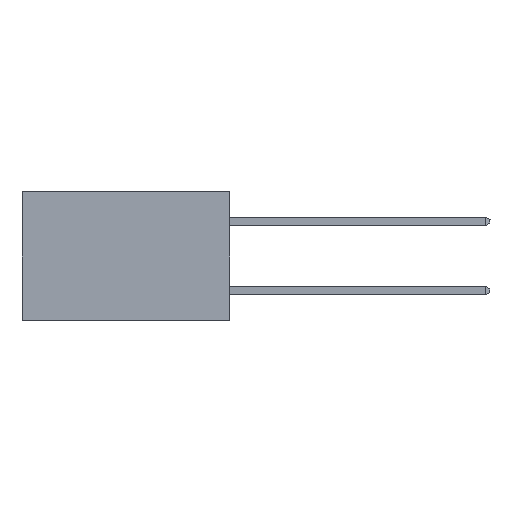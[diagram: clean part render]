
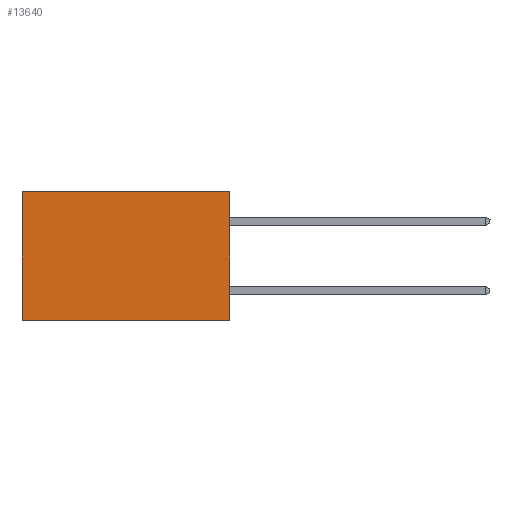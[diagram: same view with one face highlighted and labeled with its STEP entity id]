
A CAD part, left-side view. The second image highlights one B-rep face of the part: STEP entity #13640.
In plain terms, the highlighted planar face has unit normal (-1, 0, 0).
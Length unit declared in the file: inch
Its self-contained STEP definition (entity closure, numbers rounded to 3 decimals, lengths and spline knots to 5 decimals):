
#732 = DIRECTION ( 'NONE',  ( 0., 0., -1. ) ) ;
#771 = ORIENTED_EDGE ( 'NONE', *, *, #5484, .F. ) ;
#996 = VECTOR ( 'NONE', #6871, 39.37008 ) ;
#1110 = CARTESIAN_POINT ( 'NONE',  ( 0.2615, 0.6, -0.37 ) ) ;
#1194 = LINE ( 'NONE', #12657, #16201 ) ;
#1874 = CARTESIAN_POINT ( 'NONE',  ( 0.2615, 0.6, 0. ) ) ;
#2434 = PLANE ( 'NONE',  #10599 ) ;
#3651 = LINE ( 'NONE', #11792, #996 ) ;
#4259 = CARTESIAN_POINT ( 'NONE',  ( 0.2615, 0., -0.37 ) ) ;
#5484 = EDGE_CURVE ( 'NONE', #20255, #8042, #1194, .T. ) ;
#5891 = EDGE_CURVE ( 'NONE', #8042, #10948, #8633, .T. ) ;
#6721 = EDGE_CURVE ( 'NONE', #17228, #10948, #3651, .T. ) ;
#6871 = DIRECTION ( 'NONE',  ( 0., 0., -1. ) ) ;
#8042 = VERTEX_POINT ( 'NONE', #13190 ) ;
#8633 = LINE ( 'NONE', #11843, #10373 ) ;
#9214 = DIRECTION ( 'NONE',  ( 0., 1., 0. ) ) ;
#10373 = VECTOR ( 'NONE', #13558, 39.37008 ) ;
#10599 = AXIS2_PLACEMENT_3D ( 'NONE', #4259, #17211, #732 ) ;
#10783 = ORIENTED_EDGE ( 'NONE', *, *, #6721, .T. ) ;
#10948 = VERTEX_POINT ( 'NONE', #1110 ) ;
#11792 = CARTESIAN_POINT ( 'NONE',  ( 0.2615, 0.6, -0.37 ) ) ;
#11843 = CARTESIAN_POINT ( 'NONE',  ( 0.2615, 0., -0.37 ) ) ;
#11971 = FACE_OUTER_BOUND ( 'NONE', #20858, .T. ) ;
#12657 = CARTESIAN_POINT ( 'NONE',  ( 0.2615, 0., -0.37 ) ) ;
#13190 = CARTESIAN_POINT ( 'NONE',  ( 0.2615, 0., -0.37 ) ) ;
#13197 = EDGE_CURVE ( 'NONE', #20255, #17228, #15544, .T. ) ;
#13558 = DIRECTION ( 'NONE',  ( 0., 1., 0. ) ) ;
#13640 = ADVANCED_FACE ( 'NONE', ( #11971 ), #2434, .F. ) ;
#13858 = CARTESIAN_POINT ( 'NONE',  ( 0.2615, 0., 0. ) ) ;
#14012 = VECTOR ( 'NONE', #9214, 39.37008 ) ;
#15441 = CARTESIAN_POINT ( 'NONE',  ( 0.2615, 0., 0. ) ) ;
#15544 = LINE ( 'NONE', #15441, #14012 ) ;
#16201 = VECTOR ( 'NONE', #19181, 39.37008 ) ;
#17211 = DIRECTION ( 'NONE',  ( 1., 0., 0. ) ) ;
#17228 = VERTEX_POINT ( 'NONE', #1874 ) ;
#18901 = ORIENTED_EDGE ( 'NONE', *, *, #5891, .F. ) ;
#19181 = DIRECTION ( 'NONE',  ( 0., 0., -1. ) ) ;
#19499 = ORIENTED_EDGE ( 'NONE', *, *, #13197, .T. ) ;
#20255 = VERTEX_POINT ( 'NONE', #13858 ) ;
#20858 = EDGE_LOOP ( 'NONE', ( #10783, #18901, #771, #19499 ) ) ;
